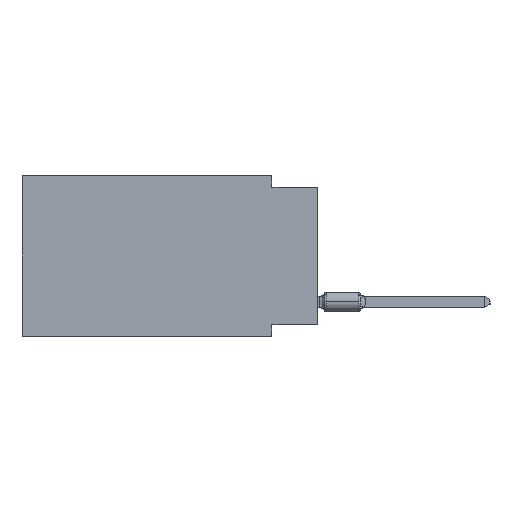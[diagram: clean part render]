
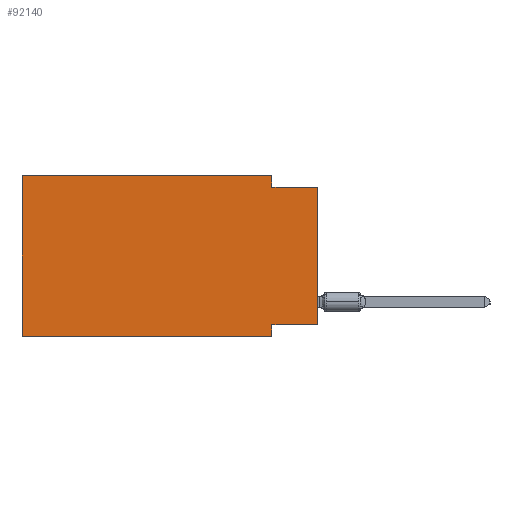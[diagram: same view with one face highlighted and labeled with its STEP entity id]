
A CAD part, left-side view. The second image highlights one B-rep face of the part: STEP entity #92140.
In plain terms, the highlighted planar face has unit normal (-1, 0, 0).
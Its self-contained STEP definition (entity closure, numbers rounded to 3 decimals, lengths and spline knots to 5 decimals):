
#233 = ORIENTED_EDGE ( 'NONE', *, *, #56091, .T. ) ;
#290 = CARTESIAN_POINT ( 'NONE',  ( 0., 0., -0.025 ) ) ;
#555 = VECTOR ( 'NONE', #5594, 39.37008 ) ;
#1946 = VECTOR ( 'NONE', #13767, 39.37008 ) ;
#3953 = EDGE_CURVE ( 'NONE', #29246, #12978, #72920, .T. ) ;
#4510 = CARTESIAN_POINT ( 'NONE',  ( 0., 0.645, 0. ) ) ;
#5594 = DIRECTION ( 'NONE',  ( 0., -1., 0. ) ) ;
#7715 = EDGE_CURVE ( 'NONE', #88822, #40666, #36131, .T. ) ;
#12572 = CARTESIAN_POINT ( 'NONE',  ( 0., 0.1, -0.35 ) ) ;
#12978 = VERTEX_POINT ( 'NONE', #81371 ) ;
#13767 = DIRECTION ( 'NONE',  ( 0., 0., 1. ) ) ;
#13859 = VERTEX_POINT ( 'NONE', #105841 ) ;
#15714 = DIRECTION ( 'NONE',  ( 0., 0., 1. ) ) ;
#16112 = CARTESIAN_POINT ( 'NONE',  ( 0., 0., -0.325 ) ) ;
#18115 = DIRECTION ( 'NONE',  ( 1., 0., 0. ) ) ;
#18792 = EDGE_LOOP ( 'NONE', ( #21022, #55421, #48418, #74847, #71617, #233, #54785, #93896 ) ) ;
#20523 = CARTESIAN_POINT ( 'NONE',  ( 0., 0.1, 0. ) ) ;
#21022 = ORIENTED_EDGE ( 'NONE', *, *, #99694, .T. ) ;
#22681 = LINE ( 'NONE', #63391, #1946 ) ;
#26386 = AXIS2_PLACEMENT_3D ( 'NONE', #84479, #18115, #52112 ) ;
#29246 = VERTEX_POINT ( 'NONE', #70363 ) ;
#33946 = DIRECTION ( 'NONE',  ( 0., -1., 0. ) ) ;
#35115 = DIRECTION ( 'NONE',  ( 0., 1., 0. ) ) ;
#36131 = LINE ( 'NONE', #41867, #102283 ) ;
#40666 = VERTEX_POINT ( 'NONE', #4510 ) ;
#41867 = CARTESIAN_POINT ( 'NONE',  ( 0., 0.645, 0. ) ) ;
#43869 = VECTOR ( 'NONE', #58792, 39.37008 ) ;
#44021 = CARTESIAN_POINT ( 'NONE',  ( 0., 0., -0.325 ) ) ;
#44743 = VERTEX_POINT ( 'NONE', #69206 ) ;
#46575 = DIRECTION ( 'NONE',  ( 0., 0., -1. ) ) ;
#47958 = LINE ( 'NONE', #89793, #555 ) ;
#48418 = ORIENTED_EDGE ( 'NONE', *, *, #3953, .F. ) ;
#49384 = EDGE_CURVE ( 'NONE', #44743, #13859, #97330, .T. ) ;
#51221 = CARTESIAN_POINT ( 'NONE',  ( 0., 0.645, 0. ) ) ;
#52112 = DIRECTION ( 'NONE',  ( 0., 0., -1. ) ) ;
#54785 = ORIENTED_EDGE ( 'NONE', *, *, #49384, .F. ) ;
#55421 = ORIENTED_EDGE ( 'NONE', *, *, #107803, .F. ) ;
#56091 = EDGE_CURVE ( 'NONE', #88822, #13859, #47958, .T. ) ;
#56169 = DIRECTION ( 'NONE',  ( 0., 0., -1. ) ) ;
#58792 = DIRECTION ( 'NONE',  ( 0., -1., 0. ) ) ;
#62167 = EDGE_CURVE ( 'NONE', #40666, #29246, #102519, .T. ) ;
#63391 = CARTESIAN_POINT ( 'NONE',  ( 0., 0., 0. ) ) ;
#64785 = VERTEX_POINT ( 'NONE', #16112 ) ;
#66625 = LINE ( 'NONE', #107899, #43869 ) ;
#69206 = CARTESIAN_POINT ( 'NONE',  ( 0., 0.1, -0.325 ) ) ;
#70363 = CARTESIAN_POINT ( 'NONE',  ( 0., 0.1, 0. ) ) ;
#71617 = ORIENTED_EDGE ( 'NONE', *, *, #7715, .F. ) ;
#72276 = VECTOR ( 'NONE', #35115, 39.37008 ) ;
#72920 = LINE ( 'NONE', #20523, #107683 ) ;
#74847 = ORIENTED_EDGE ( 'NONE', *, *, #62167, .F. ) ;
#77636 = CARTESIAN_POINT ( 'NONE',  ( 0., 0.645, -0.35 ) ) ;
#81371 = CARTESIAN_POINT ( 'NONE',  ( 0., 0.1, -0.025 ) ) ;
#84479 = CARTESIAN_POINT ( 'NONE',  ( 0., 0.645, 0. ) ) ;
#85334 = VERTEX_POINT ( 'NONE', #290 ) ;
#85877 = LINE ( 'NONE', #44021, #72276 ) ;
#88822 = VERTEX_POINT ( 'NONE', #77636 ) ;
#89179 = EDGE_CURVE ( 'NONE', #64785, #44743, #85877, .T. ) ;
#89749 = VECTOR ( 'NONE', #46575, 39.37008 ) ;
#89793 = CARTESIAN_POINT ( 'NONE',  ( 0., 0.645, -0.35 ) ) ;
#92140 = ADVANCED_FACE ( 'NONE', ( #94487 ), #110122, .F. ) ;
#93896 = ORIENTED_EDGE ( 'NONE', *, *, #89179, .F. ) ;
#94487 = FACE_OUTER_BOUND ( 'NONE', #18792, .T. ) ;
#97330 = LINE ( 'NONE', #12572, #89749 ) ;
#99459 = VECTOR ( 'NONE', #33946, 39.37008 ) ;
#99694 = EDGE_CURVE ( 'NONE', #64785, #85334, #22681, .T. ) ;
#102283 = VECTOR ( 'NONE', #15714, 39.37008 ) ;
#102519 = LINE ( 'NONE', #51221, #99459 ) ;
#105841 = CARTESIAN_POINT ( 'NONE',  ( 0., 0.1, -0.35 ) ) ;
#107683 = VECTOR ( 'NONE', #56169, 39.37008 ) ;
#107803 = EDGE_CURVE ( 'NONE', #12978, #85334, #66625, .T. ) ;
#107899 = CARTESIAN_POINT ( 'NONE',  ( 0., 0., -0.025 ) ) ;
#110122 = PLANE ( 'NONE',  #26386 ) ;
